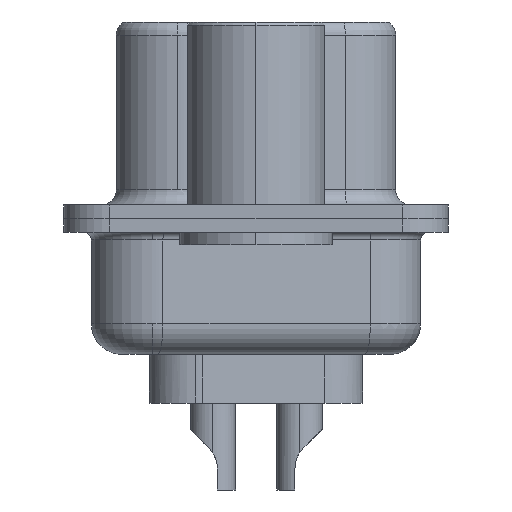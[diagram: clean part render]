
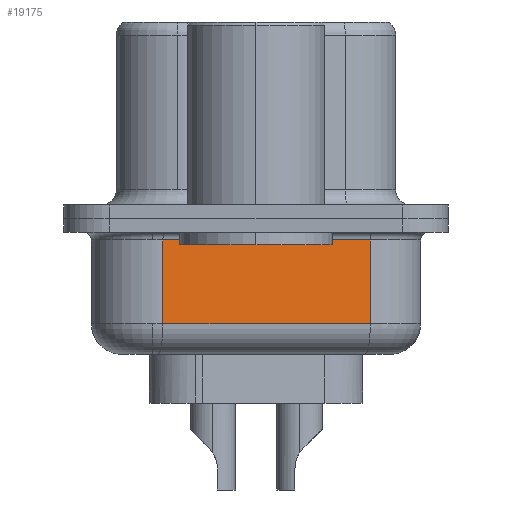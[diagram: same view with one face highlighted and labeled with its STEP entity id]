
A CAD part, left-side view. The second image highlights one B-rep face of the part: STEP entity #19175.
In plain terms, the highlighted planar face has unit normal (-0.985, -0.174, 0).
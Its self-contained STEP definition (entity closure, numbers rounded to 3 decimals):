
#442 = LINE ( 'NONE', #4994, #562 ) ;
#499 = CARTESIAN_POINT ( 'NONE',  ( 2.89, 3.053, -4.45 ) ) ;
#562 = VECTOR ( 'NONE', #7976, 1000. ) ;
#637 = FACE_OUTER_BOUND ( 'NONE', #1066, .T. ) ;
#777 = CARTESIAN_POINT ( 'NONE',  ( 2.89, 3.053, -0.7 ) ) ;
#1066 = EDGE_LOOP ( 'NONE', ( #17199, #13608, #8036, #6159 ) ) ;
#2186 = EDGE_CURVE ( 'NONE', #4032, #5871, #17892, .T. ) ;
#2321 = PLANE ( 'NONE',  #9846 ) ;
#2751 = DIRECTION ( 'NONE',  ( 0.174, -0.985, 0. ) ) ;
#4032 = VERTEX_POINT ( 'NONE', #10207 ) ;
#4994 = CARTESIAN_POINT ( 'NONE',  ( 2.89, 3.053, -0.7 ) ) ;
#5641 = VERTEX_POINT ( 'NONE', #8812 ) ;
#5653 = VECTOR ( 'NONE', #17026, 1000. ) ;
#5871 = VERTEX_POINT ( 'NONE', #11094 ) ;
#6159 = ORIENTED_EDGE ( 'NONE', *, *, #15155, .T. ) ;
#6637 = VECTOR ( 'NONE', #11276, 1000. ) ;
#7976 = DIRECTION ( 'NONE',  ( -0.174, 0.985, 0. ) ) ;
#8036 = ORIENTED_EDGE ( 'NONE', *, *, #16915, .T. ) ;
#8375 = CARTESIAN_POINT ( 'NONE',  ( 2.89, 3.053, -4.45 ) ) ;
#8812 = CARTESIAN_POINT ( 'NONE',  ( 4.089, -3.747, -0.7 ) ) ;
#8906 = CARTESIAN_POINT ( 'NONE',  ( 2.89, 3.053, -3.45 ) ) ;
#9846 = AXIS2_PLACEMENT_3D ( 'NONE', #8375, #12948, #19058 ) ;
#10207 = CARTESIAN_POINT ( 'NONE',  ( 2.89, 3.053, -3.45 ) ) ;
#11094 = CARTESIAN_POINT ( 'NONE',  ( 4.089, -3.747, -3.45 ) ) ;
#11276 = DIRECTION ( 'NONE',  ( 0., 0., 1. ) ) ;
#12948 = DIRECTION ( 'NONE',  ( 0.985, 0.174, 0. ) ) ;
#13608 = ORIENTED_EDGE ( 'NONE', *, *, #2186, .T. ) ;
#14247 = CARTESIAN_POINT ( 'NONE',  ( 4.089, -3.747, -4.45 ) ) ;
#15155 = EDGE_CURVE ( 'NONE', #5641, #15991, #442, .T. ) ;
#15816 = EDGE_CURVE ( 'NONE', #4032, #15991, #17230, .T. ) ;
#15991 = VERTEX_POINT ( 'NONE', #777 ) ;
#16915 = EDGE_CURVE ( 'NONE', #5871, #5641, #17654, .T. ) ;
#17026 = DIRECTION ( 'NONE',  ( 0., 0., 1. ) ) ;
#17199 = ORIENTED_EDGE ( 'NONE', *, *, #15816, .F. ) ;
#17230 = LINE ( 'NONE', #499, #5653 ) ;
#17654 = LINE ( 'NONE', #14247, #6637 ) ;
#17892 = LINE ( 'NONE', #8906, #18828 ) ;
#18828 = VECTOR ( 'NONE', #2751, 1000. ) ;
#19058 = DIRECTION ( 'NONE',  ( -0.174, 0.985, 0. ) ) ;
#19175 = ADVANCED_FACE ( 'NONE', ( #637 ), #2321, .F. ) ;
